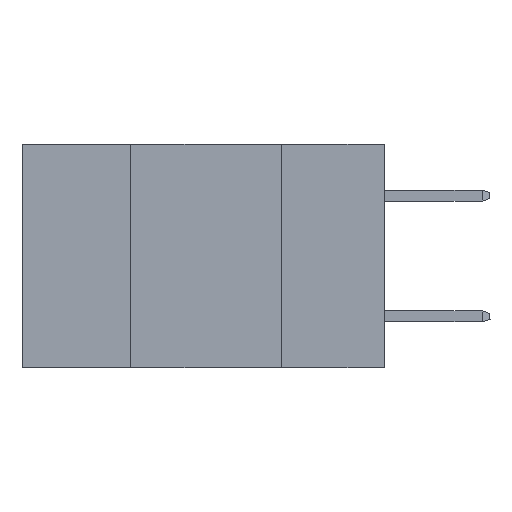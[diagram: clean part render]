
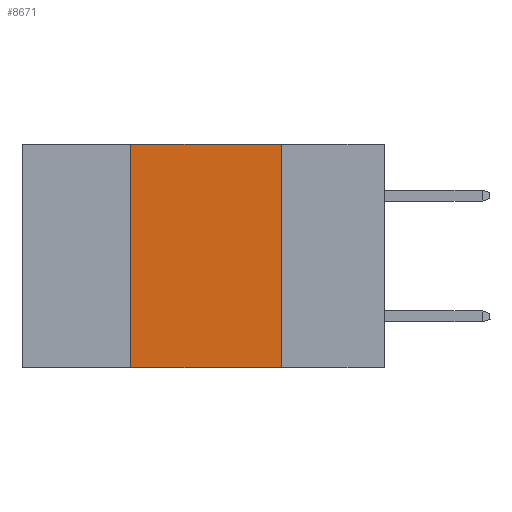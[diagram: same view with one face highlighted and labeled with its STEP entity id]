
A CAD part, left-side view. The second image highlights one B-rep face of the part: STEP entity #8671.
In plain terms, the highlighted planar face has unit normal (-1, 0, 0).
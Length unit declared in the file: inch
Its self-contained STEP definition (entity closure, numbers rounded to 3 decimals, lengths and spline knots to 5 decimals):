
#831 = VERTEX_POINT ( 'NONE', #6322 ) ;
#1421 = ORIENTED_EDGE ( 'NONE', *, *, #15748, .T. ) ;
#1617 = VECTOR ( 'NONE', #17090, 39.37008 ) ;
#1636 = VERTEX_POINT ( 'NONE', #9588 ) ;
#1669 = EDGE_LOOP ( 'NONE', ( #8636, #12691, #7061, #1421 ) ) ;
#1890 = PLANE ( 'NONE',  #7757 ) ;
#3317 = DIRECTION ( 'NONE',  ( 1., 0., 0. ) ) ;
#3601 = EDGE_CURVE ( 'NONE', #13946, #16823, #17775, .T. ) ;
#4472 = VECTOR ( 'NONE', #16027, 39.37008 ) ;
#4946 = CARTESIAN_POINT ( 'NONE',  ( 0., 0.6, -0.37 ) ) ;
#6150 = LINE ( 'NONE', #4946, #17202 ) ;
#6322 = CARTESIAN_POINT ( 'NONE',  ( 0., 0.42, 0. ) ) ;
#6437 = DIRECTION ( 'NONE',  ( 0., -1., 0. ) ) ;
#7006 = CARTESIAN_POINT ( 'NONE',  ( 0., 0.6, 0. ) ) ;
#7061 = ORIENTED_EDGE ( 'NONE', *, *, #11875, .F. ) ;
#7256 = FACE_OUTER_BOUND ( 'NONE', #1669, .T. ) ;
#7757 = AXIS2_PLACEMENT_3D ( 'NONE', #11999, #3317, #13476 ) ;
#8347 = EDGE_CURVE ( 'NONE', #831, #13946, #12697, .T. ) ;
#8636 = ORIENTED_EDGE ( 'NONE', *, *, #3601, .F. ) ;
#8671 = ADVANCED_FACE ( 'NONE', ( #7256 ), #1890, .F. ) ;
#9588 = CARTESIAN_POINT ( 'NONE',  ( 0., 0.42, -0.37 ) ) ;
#9605 = DIRECTION ( 'NONE',  ( 0., 0., -1. ) ) ;
#9626 = CARTESIAN_POINT ( 'NONE',  ( 0., 0.17, -0.37 ) ) ;
#11875 = EDGE_CURVE ( 'NONE', #1636, #831, #12215, .T. ) ;
#11999 = CARTESIAN_POINT ( 'NONE',  ( 0., 0.6, 0. ) ) ;
#12215 = LINE ( 'NONE', #14589, #4472 ) ;
#12691 = ORIENTED_EDGE ( 'NONE', *, *, #8347, .F. ) ;
#12697 = LINE ( 'NONE', #7006, #1617 ) ;
#13341 = CARTESIAN_POINT ( 'NONE',  ( 0., 0.17, 0. ) ) ;
#13476 = DIRECTION ( 'NONE',  ( 0., 0., -1. ) ) ;
#13580 = VECTOR ( 'NONE', #9605, 39.37008 ) ;
#13946 = VERTEX_POINT ( 'NONE', #13341 ) ;
#14589 = CARTESIAN_POINT ( 'NONE',  ( 0., 0.42, -0.37 ) ) ;
#15748 = EDGE_CURVE ( 'NONE', #1636, #16823, #6150, .T. ) ;
#16027 = DIRECTION ( 'NONE',  ( 0., 0., 1. ) ) ;
#16823 = VERTEX_POINT ( 'NONE', #17230 ) ;
#17090 = DIRECTION ( 'NONE',  ( 0., -1., 0. ) ) ;
#17202 = VECTOR ( 'NONE', #6437, 39.37008 ) ;
#17230 = CARTESIAN_POINT ( 'NONE',  ( 0., 0.17, -0.37 ) ) ;
#17775 = LINE ( 'NONE', #9626, #13580 ) ;
